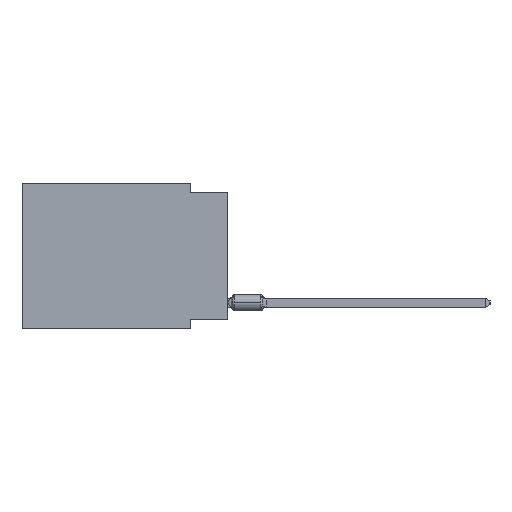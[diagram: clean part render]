
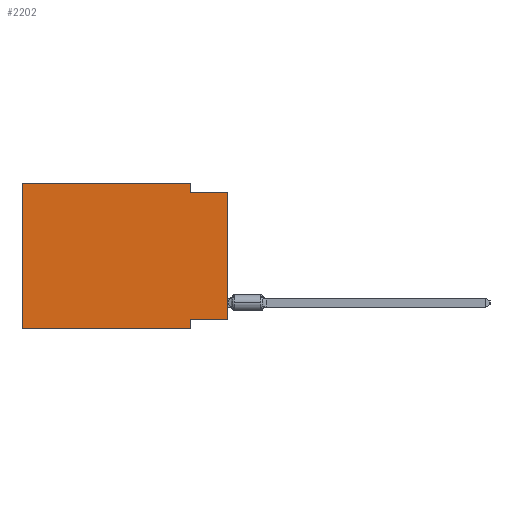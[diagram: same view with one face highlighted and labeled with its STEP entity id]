
A CAD part, left-side view. The second image highlights one B-rep face of the part: STEP entity #2202.
In plain terms, the highlighted planar face has unit normal (-1, 0, 0).
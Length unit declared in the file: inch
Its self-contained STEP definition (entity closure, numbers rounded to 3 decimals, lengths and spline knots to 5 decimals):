
#1086 = VERTEX_POINT ( 'NONE', #12233 ) ;
#1557 = CARTESIAN_POINT ( 'NONE',  ( 0., 0.1, -0.39 ) ) ;
#1950 = EDGE_LOOP ( 'NONE', ( #8310, #16998, #10714, #15815, #17448, #11642, #12866, #19251 ) ) ;
#2202 = ADVANCED_FACE ( 'NONE', ( #17419 ), #29543, .F. ) ;
#3479 = VERTEX_POINT ( 'NONE', #5943 ) ;
#4157 = VECTOR ( 'NONE', #24703, 39.37008 ) ;
#5943 = CARTESIAN_POINT ( 'NONE',  ( 0., 0., -0.025 ) ) ;
#8310 = ORIENTED_EDGE ( 'NONE', *, *, #22632, .T. ) ;
#9087 = LINE ( 'NONE', #16368, #49087 ) ;
#9147 = VERTEX_POINT ( 'NONE', #9749 ) ;
#9395 = DIRECTION ( 'NONE',  ( 0., 0., 1. ) ) ;
#9749 = CARTESIAN_POINT ( 'NONE',  ( 0., 0.1, -0.39 ) ) ;
#10208 = LINE ( 'NONE', #29856, #14776 ) ;
#10714 = ORIENTED_EDGE ( 'NONE', *, *, #45267, .F. ) ;
#10788 = DIRECTION ( 'NONE',  ( 0., -1., 0. ) ) ;
#11642 = ORIENTED_EDGE ( 'NONE', *, *, #39150, .T. ) ;
#11717 = VERTEX_POINT ( 'NONE', #47358 ) ;
#12233 = CARTESIAN_POINT ( 'NONE',  ( 0., 0.1, -0.025 ) ) ;
#12807 = VERTEX_POINT ( 'NONE', #14935 ) ;
#12866 = ORIENTED_EDGE ( 'NONE', *, *, #34461, .F. ) ;
#13412 = LINE ( 'NONE', #24514, #46620 ) ;
#13619 = LINE ( 'NONE', #40606, #44043 ) ;
#14776 = VECTOR ( 'NONE', #25570, 39.37008 ) ;
#14935 = CARTESIAN_POINT ( 'NONE',  ( 0., 0., -0.365 ) ) ;
#15815 = ORIENTED_EDGE ( 'NONE', *, *, #29533, .F. ) ;
#16368 = CARTESIAN_POINT ( 'NONE',  ( 0., 0., -0.025 ) ) ;
#16998 = ORIENTED_EDGE ( 'NONE', *, *, #23028, .F. ) ;
#17359 = LINE ( 'NONE', #1557, #30680 ) ;
#17419 = FACE_OUTER_BOUND ( 'NONE', #1950, .T. ) ;
#17448 = ORIENTED_EDGE ( 'NONE', *, *, #28216, .F. ) ;
#17461 = CARTESIAN_POINT ( 'NONE',  ( 0., 0.55, 0. ) ) ;
#18709 = CARTESIAN_POINT ( 'NONE',  ( 0., 0.1, 0. ) ) ;
#19251 = ORIENTED_EDGE ( 'NONE', *, *, #34437, .F. ) ;
#19494 = VERTEX_POINT ( 'NONE', #17461 ) ;
#20903 = DIRECTION ( 'NONE',  ( 0., 0., -1. ) ) ;
#22632 = EDGE_CURVE ( 'NONE', #12807, #3479, #13412, .T. ) ;
#23028 = EDGE_CURVE ( 'NONE', #1086, #3479, #9087, .T. ) ;
#24514 = CARTESIAN_POINT ( 'NONE',  ( 0., 0., 0. ) ) ;
#24703 = DIRECTION ( 'NONE',  ( 0., 1., 0. ) ) ;
#25508 = DIRECTION ( 'NONE',  ( 1., 0., 0. ) ) ;
#25570 = DIRECTION ( 'NONE',  ( 0., 0., 1. ) ) ;
#25813 = AXIS2_PLACEMENT_3D ( 'NONE', #26010, #25508, #36615 ) ;
#26010 = CARTESIAN_POINT ( 'NONE',  ( 0., 0.55, 0. ) ) ;
#26576 = VERTEX_POINT ( 'NONE', #39380 ) ;
#26679 = DIRECTION ( 'NONE',  ( 0., -1., 0. ) ) ;
#28216 = EDGE_CURVE ( 'NONE', #26576, #19494, #10208, .T. ) ;
#28952 = CARTESIAN_POINT ( 'NONE',  ( 0., 0.55, -0.39 ) ) ;
#29533 = EDGE_CURVE ( 'NONE', #19494, #40151, #42290, .T. ) ;
#29543 = PLANE ( 'NONE',  #25813 ) ;
#29856 = CARTESIAN_POINT ( 'NONE',  ( 0., 0.55, 0. ) ) ;
#30680 = VECTOR ( 'NONE', #20903, 39.37008 ) ;
#32497 = LINE ( 'NONE', #37047, #4157 ) ;
#34239 = CARTESIAN_POINT ( 'NONE',  ( 0., 0.55, 0. ) ) ;
#34437 = EDGE_CURVE ( 'NONE', #12807, #11717, #32497, .T. ) ;
#34461 = EDGE_CURVE ( 'NONE', #11717, #9147, #17359, .T. ) ;
#35381 = DIRECTION ( 'NONE',  ( 0., 0., -1. ) ) ;
#35556 = DIRECTION ( 'NONE',  ( 0., -1., 0. ) ) ;
#35715 = VECTOR ( 'NONE', #10788, 39.37008 ) ;
#35736 = VECTOR ( 'NONE', #26679, 39.37008 ) ;
#36615 = DIRECTION ( 'NONE',  ( 0., 0., -1. ) ) ;
#37047 = CARTESIAN_POINT ( 'NONE',  ( 0., 0., -0.365 ) ) ;
#39150 = EDGE_CURVE ( 'NONE', #26576, #9147, #48602, .T. ) ;
#39380 = CARTESIAN_POINT ( 'NONE',  ( 0., 0.55, -0.39 ) ) ;
#40151 = VERTEX_POINT ( 'NONE', #18709 ) ;
#40606 = CARTESIAN_POINT ( 'NONE',  ( 0., 0.1, 0. ) ) ;
#42290 = LINE ( 'NONE', #34239, #35736 ) ;
#44043 = VECTOR ( 'NONE', #35381, 39.37008 ) ;
#45267 = EDGE_CURVE ( 'NONE', #40151, #1086, #13619, .T. ) ;
#46620 = VECTOR ( 'NONE', #9395, 39.37008 ) ;
#47358 = CARTESIAN_POINT ( 'NONE',  ( 0., 0.1, -0.365 ) ) ;
#48602 = LINE ( 'NONE', #28952, #35715 ) ;
#49087 = VECTOR ( 'NONE', #35556, 39.37008 ) ;
